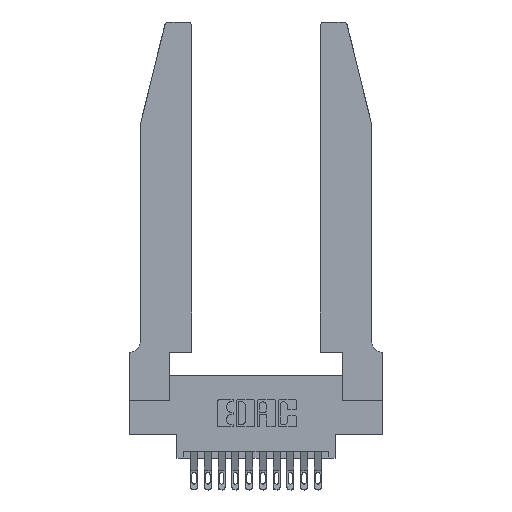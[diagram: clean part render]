
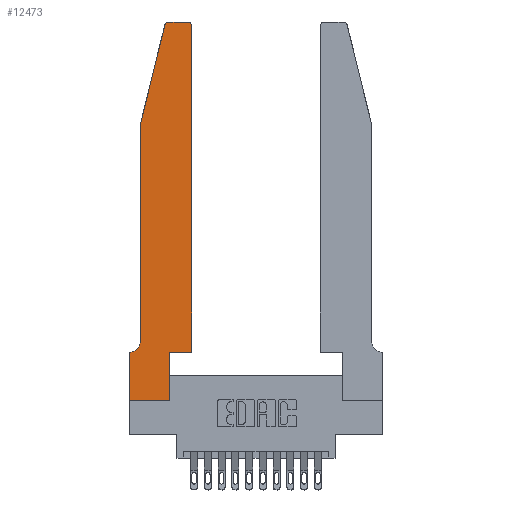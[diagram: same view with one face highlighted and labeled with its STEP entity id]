
A CAD part, top view. The second image highlights one B-rep face of the part: STEP entity #12473.
In plain terms, the highlighted planar face has unit normal (0, 0, 1).
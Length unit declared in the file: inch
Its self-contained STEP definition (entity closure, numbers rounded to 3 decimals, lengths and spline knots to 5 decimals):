
#113 = PLANE ( 'NONE',  #17271 ) ;
#208 = VECTOR ( 'NONE', #12831, 39.37008 ) ;
#268 = AXIS2_PLACEMENT_3D ( 'NONE', #8524, #4514, #5959 ) ;
#291 = LINE ( 'NONE', #16358, #9755 ) ;
#346 = VERTEX_POINT ( 'NONE', #12331 ) ;
#546 = VERTEX_POINT ( 'NONE', #1315 ) ;
#625 = ORIENTED_EDGE ( 'NONE', *, *, #5610, .T. ) ;
#823 = EDGE_CURVE ( 'NONE', #13946, #8675, #1258, .T. ) ;
#862 = FACE_OUTER_BOUND ( 'NONE', #14681, .T. ) ;
#865 = VERTEX_POINT ( 'NONE', #1126 ) ;
#1126 = CARTESIAN_POINT ( 'NONE',  ( 0.0055, 0.35, 0.37 ) ) ;
#1165 = DIRECTION ( 'NONE',  ( 1., 0., 0. ) ) ;
#1249 = CARTESIAN_POINT ( 'NONE',  ( 0.0755, 0.42, 0.37 ) ) ;
#1253 = VECTOR ( 'NONE', #17193, 39.37008 ) ;
#1258 = LINE ( 'NONE', #9111, #15142 ) ;
#1282 = CARTESIAN_POINT ( 'NONE',  ( 0.284, 2.75, 0.37 ) ) ;
#1315 = CARTESIAN_POINT ( 'NONE',  ( 0.4505, 2.72, 0.37 ) ) ;
#1706 = CARTESIAN_POINT ( 'NONE',  ( 0.4505, 0.35, 0.37 ) ) ;
#1773 = DIRECTION ( 'NONE',  ( 0., 0., -1. ) ) ;
#1971 = VERTEX_POINT ( 'NONE', #1249 ) ;
#3098 = CARTESIAN_POINT ( 'NONE',  ( 0.4205, 2.75, 0.37 ) ) ;
#3123 = DIRECTION ( 'NONE',  ( -1., 0., 0. ) ) ;
#3194 = VECTOR ( 'NONE', #13759, 39.37008 ) ;
#3664 = VERTEX_POINT ( 'NONE', #15159 ) ;
#3919 = DIRECTION ( 'NONE',  ( 1., 0., 0. ) ) ;
#3955 = EDGE_CURVE ( 'NONE', #3664, #346, #12363, .T. ) ;
#3958 = EDGE_CURVE ( 'NONE', #4390, #16903, #10427, .T. ) ;
#4390 = VERTEX_POINT ( 'NONE', #6299 ) ;
#4514 = DIRECTION ( 'NONE',  ( 0., 0., 1. ) ) ;
#4943 = VERTEX_POINT ( 'NONE', #13995 ) ;
#5063 = DIRECTION ( 'NONE',  ( 0., 0., 1. ) ) ;
#5080 = ORIENTED_EDGE ( 'NONE', *, *, #16990, .T. ) ;
#5610 = EDGE_CURVE ( 'NONE', #546, #14988, #12897, .T. ) ;
#5959 = DIRECTION ( 'NONE',  ( 1., 0., 0. ) ) ;
#6299 = CARTESIAN_POINT ( 'NONE',  ( 0.25487, 2.72718, 0.37 ) ) ;
#6431 = VECTOR ( 'NONE', #1165, 39.37008 ) ;
#6469 = CARTESIAN_POINT ( 'NONE',  ( 0., 0., 0.37 ) ) ;
#6947 = DIRECTION ( 'NONE',  ( -1., 0., 0. ) ) ;
#7347 = EDGE_CURVE ( 'NONE', #346, #13946, #13285, .T. ) ;
#7563 = CARTESIAN_POINT ( 'NONE',  ( 0.2865, 0.35, 0.37 ) ) ;
#8155 = EDGE_CURVE ( 'NONE', #16903, #1971, #16938, .T. ) ;
#8286 = CARTESIAN_POINT ( 'NONE',  ( 0., 0.35, 0.37 ) ) ;
#8524 = CARTESIAN_POINT ( 'NONE',  ( 0.4205, 2.72, 0.37 ) ) ;
#8643 = CIRCLE ( 'NONE', #10417, 0.07 ) ;
#8675 = VERTEX_POINT ( 'NONE', #14132 ) ;
#9111 = CARTESIAN_POINT ( 'NONE',  ( 0.4505, 0.35, 0.37 ) ) ;
#9394 = CARTESIAN_POINT ( 'NONE',  ( 0., 0., 0.37 ) ) ;
#9404 = ORIENTED_EDGE ( 'NONE', *, *, #3958, .T. ) ;
#9490 = EDGE_CURVE ( 'NONE', #10503, #4390, #12967, .T. ) ;
#9755 = VECTOR ( 'NONE', #6947, 39.37008 ) ;
#9801 = CARTESIAN_POINT ( 'NONE',  ( 0.0055, 0.42, 0.37 ) ) ;
#9869 = LINE ( 'NONE', #6469, #1253 ) ;
#10417 = AXIS2_PLACEMENT_3D ( 'NONE', #9801, #1773, #3123 ) ;
#10427 = LINE ( 'NONE', #10598, #17132 ) ;
#10503 = VERTEX_POINT ( 'NONE', #1282 ) ;
#10598 = CARTESIAN_POINT ( 'NONE',  ( 0.0755, 2., 0.37 ) ) ;
#10859 = EDGE_CURVE ( 'NONE', #14988, #10503, #291, .T. ) ;
#10910 = VECTOR ( 'NONE', #14495, 39.37008 ) ;
#11280 = ORIENTED_EDGE ( 'NONE', *, *, #8155, .T. ) ;
#11389 = CARTESIAN_POINT ( 'NONE',  ( 0.2865, 0.35, 0.37 ) ) ;
#11398 = VECTOR ( 'NONE', #11801, 39.37008 ) ;
#11591 = AXIS2_PLACEMENT_3D ( 'NONE', #14513, #5063, #17129 ) ;
#11801 = DIRECTION ( 'NONE',  ( -1., 0., 0. ) ) ;
#12317 = DIRECTION ( 'NONE',  ( 0., 0., 1. ) ) ;
#12331 = CARTESIAN_POINT ( 'NONE',  ( 0.2865, 0., 0.37 ) ) ;
#12363 = LINE ( 'NONE', #9394, #6431 ) ;
#12473 = ADVANCED_FACE ( 'NONE', ( #862 ), #113, .T. ) ;
#12570 = EDGE_CURVE ( 'NONE', #8675, #546, #16199, .T. ) ;
#12640 = EDGE_CURVE ( 'NONE', #1971, #865, #8643, .T. ) ;
#12831 = DIRECTION ( 'NONE',  ( 0., 1., 0. ) ) ;
#12897 = CIRCLE ( 'NONE', #268, 0.03 ) ;
#12967 = CIRCLE ( 'NONE', #11591, 0.03 ) ;
#13028 = ORIENTED_EDGE ( 'NONE', *, *, #12570, .T. ) ;
#13285 = LINE ( 'NONE', #11389, #208 ) ;
#13299 = DIRECTION ( 'NONE',  ( -0.239, -0.971, 0. ) ) ;
#13408 = EDGE_CURVE ( 'NONE', #4943, #3664, #9869, .T. ) ;
#13711 = DIRECTION ( 'NONE',  ( 1., 0., 0. ) ) ;
#13759 = DIRECTION ( 'NONE',  ( 0., 1., 0. ) ) ;
#13946 = VERTEX_POINT ( 'NONE', #7563 ) ;
#13995 = CARTESIAN_POINT ( 'NONE',  ( 0., 0.35, 0.37 ) ) ;
#14005 = CARTESIAN_POINT ( 'NONE',  ( 0.0755, 2., 0.37 ) ) ;
#14132 = CARTESIAN_POINT ( 'NONE',  ( 0.4505, 0.35, 0.37 ) ) ;
#14495 = DIRECTION ( 'NONE',  ( 0., -1., 0. ) ) ;
#14513 = CARTESIAN_POINT ( 'NONE',  ( 0.284, 2.72, 0.37 ) ) ;
#14605 = ORIENTED_EDGE ( 'NONE', *, *, #7347, .T. ) ;
#14644 = ORIENTED_EDGE ( 'NONE', *, *, #3955, .T. ) ;
#14681 = EDGE_LOOP ( 'NONE', ( #16951, #15815, #9404, #11280, #15665, #5080, #15383, #14644, #14605, #17373, #13028, #625 ) ) ;
#14988 = VERTEX_POINT ( 'NONE', #3098 ) ;
#15142 = VECTOR ( 'NONE', #3919, 39.37008 ) ;
#15159 = CARTESIAN_POINT ( 'NONE',  ( 0., 0., 0.37 ) ) ;
#15383 = ORIENTED_EDGE ( 'NONE', *, *, #13408, .T. ) ;
#15543 = LINE ( 'NONE', #15613, #11398 ) ;
#15613 = CARTESIAN_POINT ( 'NONE',  ( 0.0755, 0.35, 0.37 ) ) ;
#15665 = ORIENTED_EDGE ( 'NONE', *, *, #12640, .T. ) ;
#15815 = ORIENTED_EDGE ( 'NONE', *, *, #9490, .T. ) ;
#16199 = LINE ( 'NONE', #1706, #3194 ) ;
#16358 = CARTESIAN_POINT ( 'NONE',  ( 0.2605, 2.75, 0.37 ) ) ;
#16903 = VERTEX_POINT ( 'NONE', #14005 ) ;
#16938 = LINE ( 'NONE', #16988, #10910 ) ;
#16951 = ORIENTED_EDGE ( 'NONE', *, *, #10859, .T. ) ;
#16988 = CARTESIAN_POINT ( 'NONE',  ( 0.0755, 2., 0.37 ) ) ;
#16990 = EDGE_CURVE ( 'NONE', #865, #4943, #15543, .T. ) ;
#17129 = DIRECTION ( 'NONE',  ( 1., 0., 0. ) ) ;
#17132 = VECTOR ( 'NONE', #13299, 39.37008 ) ;
#17193 = DIRECTION ( 'NONE',  ( 0., -1., 0. ) ) ;
#17271 = AXIS2_PLACEMENT_3D ( 'NONE', #8286, #12317, #13711 ) ;
#17373 = ORIENTED_EDGE ( 'NONE', *, *, #823, .T. ) ;
